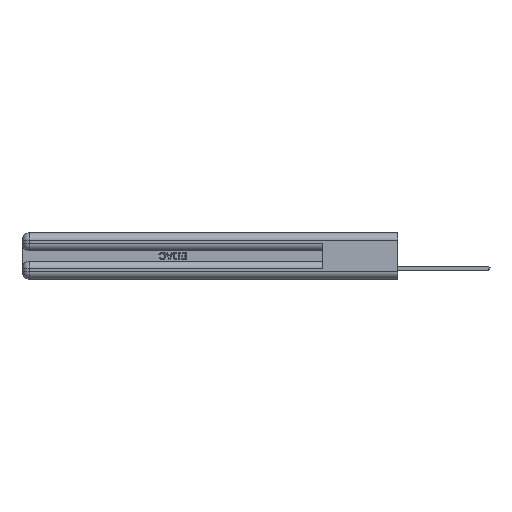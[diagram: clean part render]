
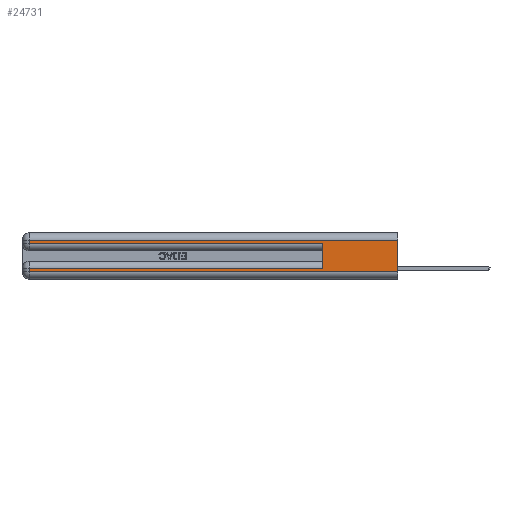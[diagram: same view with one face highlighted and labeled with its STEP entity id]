
A CAD part, left-side view. The second image highlights one B-rep face of the part: STEP entity #24731.
In plain terms, the highlighted planar face has unit normal (-1, 0, 0).
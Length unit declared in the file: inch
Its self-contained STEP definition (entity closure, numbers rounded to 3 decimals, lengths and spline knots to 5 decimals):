
#61 = EDGE_CURVE ( 'NONE', #3752, #46846, #10816, .T. ) ;
#326 = CARTESIAN_POINT ( 'NONE',  ( 0., 0., 0.31 ) ) ;
#352 = ORIENTED_EDGE ( 'NONE', *, *, #61, .T. ) ;
#1134 = AXIS2_PLACEMENT_3D ( 'NONE', #9378, #42644, #31927 ) ;
#1310 = DIRECTION ( 'NONE',  ( 0., -1., 0. ) ) ;
#1740 = VECTOR ( 'NONE', #8494, 39.37008 ) ;
#2033 = PLANE ( 'NONE',  #1134 ) ;
#3752 = VERTEX_POINT ( 'NONE', #38938 ) ;
#4401 = CARTESIAN_POINT ( 'NONE',  ( 0., 0., 0.085 ) ) ;
#5193 = CARTESIAN_POINT ( 'NONE',  ( 0., 2.94, 0.06 ) ) ;
#8428 = CARTESIAN_POINT ( 'NONE',  ( 0., 0., 0.37 ) ) ;
#8494 = DIRECTION ( 'NONE',  ( 0., 1., 0. ) ) ;
#8596 = DIRECTION ( 'NONE',  ( 0., 0., -1. ) ) ;
#8716 = ORIENTED_EDGE ( 'NONE', *, *, #35831, .T. ) ;
#8959 = CARTESIAN_POINT ( 'NONE',  ( 0., 0.6, 0.145 ) ) ;
#9278 = DIRECTION ( 'NONE',  ( 0., 0., 1. ) ) ;
#9378 = CARTESIAN_POINT ( 'NONE',  ( 0., 0., 0.37 ) ) ;
#9551 = LINE ( 'NONE', #8428, #48079 ) ;
#10088 = LINE ( 'NONE', #14343, #26941 ) ;
#10816 = LINE ( 'NONE', #44709, #32414 ) ;
#11640 = FACE_OUTER_BOUND ( 'NONE', #23321, .T. ) ;
#12915 = ORIENTED_EDGE ( 'NONE', *, *, #38808, .T. ) ;
#12947 = VECTOR ( 'NONE', #1310, 39.37008 ) ;
#13394 = VECTOR ( 'NONE', #22491, 39.37008 ) ;
#14343 = CARTESIAN_POINT ( 'NONE',  ( 0., 2.94, 0.37 ) ) ;
#15119 = VERTEX_POINT ( 'NONE', #23335 ) ;
#17437 = VERTEX_POINT ( 'NONE', #38803 ) ;
#18288 = DIRECTION ( 'NONE',  ( 0., 0., -1. ) ) ;
#22491 = DIRECTION ( 'NONE',  ( 0., -1., 0. ) ) ;
#22713 = ORIENTED_EDGE ( 'NONE', *, *, #33896, .F. ) ;
#23321 = EDGE_LOOP ( 'NONE', ( #37339, #12915, #352, #38529, #22713, #45326, #8716, #40803 ) ) ;
#23335 = CARTESIAN_POINT ( 'NONE',  ( 0., 2.94, 0.085 ) ) ;
#23594 = EDGE_CURVE ( 'NONE', #42428, #37310, #27506, .T. ) ;
#24731 = ADVANCED_FACE ( 'NONE', ( #11640 ), #2033, .F. ) ;
#25144 = VERTEX_POINT ( 'NONE', #41375 ) ;
#25438 = VECTOR ( 'NONE', #9278, 39.37008 ) ;
#26444 = DIRECTION ( 'NONE',  ( 0., 1., 0. ) ) ;
#26491 = CARTESIAN_POINT ( 'NONE',  ( 0., 0., 0.06 ) ) ;
#26941 = VECTOR ( 'NONE', #40425, 39.37008 ) ;
#27184 = EDGE_CURVE ( 'NONE', #25144, #15119, #45492, .T. ) ;
#27506 = LINE ( 'NONE', #36978, #12947 ) ;
#27802 = EDGE_CURVE ( 'NONE', #46846, #17437, #39647, .T. ) ;
#29089 = CARTESIAN_POINT ( 'NONE',  ( 0., 0., 0.285 ) ) ;
#30854 = EDGE_CURVE ( 'NONE', #34328, #37310, #9551, .T. ) ;
#31927 = DIRECTION ( 'NONE',  ( 0., 0., -1. ) ) ;
#32414 = VECTOR ( 'NONE', #18288, 39.37008 ) ;
#33756 = VECTOR ( 'NONE', #26444, 39.37008 ) ;
#33896 = EDGE_CURVE ( 'NONE', #25144, #17437, #41257, .T. ) ;
#34328 = VERTEX_POINT ( 'NONE', #38257 ) ;
#35831 = EDGE_CURVE ( 'NONE', #15119, #42428, #10088, .T. ) ;
#36978 = CARTESIAN_POINT ( 'NONE',  ( 0., 0., 0.06 ) ) ;
#37193 = CARTESIAN_POINT ( 'NONE',  ( 0., 2.94, 0.285 ) ) ;
#37310 = VERTEX_POINT ( 'NONE', #26491 ) ;
#37339 = ORIENTED_EDGE ( 'NONE', *, *, #30854, .F. ) ;
#38257 = CARTESIAN_POINT ( 'NONE',  ( 0., 0., 0.31 ) ) ;
#38529 = ORIENTED_EDGE ( 'NONE', *, *, #27802, .T. ) ;
#38803 = CARTESIAN_POINT ( 'NONE',  ( 0., 0.6, 0.285 ) ) ;
#38808 = EDGE_CURVE ( 'NONE', #34328, #3752, #46564, .T. ) ;
#38938 = CARTESIAN_POINT ( 'NONE',  ( 0., 2.94, 0.31 ) ) ;
#39647 = LINE ( 'NONE', #29089, #13394 ) ;
#40425 = DIRECTION ( 'NONE',  ( 0., 0., -1. ) ) ;
#40803 = ORIENTED_EDGE ( 'NONE', *, *, #23594, .T. ) ;
#41257 = LINE ( 'NONE', #8959, #25438 ) ;
#41375 = CARTESIAN_POINT ( 'NONE',  ( 0., 0.6, 0.085 ) ) ;
#42428 = VERTEX_POINT ( 'NONE', #5193 ) ;
#42644 = DIRECTION ( 'NONE',  ( 1., 0., 0. ) ) ;
#44709 = CARTESIAN_POINT ( 'NONE',  ( 0., 2.94, 0.37 ) ) ;
#45326 = ORIENTED_EDGE ( 'NONE', *, *, #27184, .T. ) ;
#45492 = LINE ( 'NONE', #4401, #1740 ) ;
#46564 = LINE ( 'NONE', #326, #33756 ) ;
#46846 = VERTEX_POINT ( 'NONE', #37193 ) ;
#48079 = VECTOR ( 'NONE', #8596, 39.37008 ) ;
